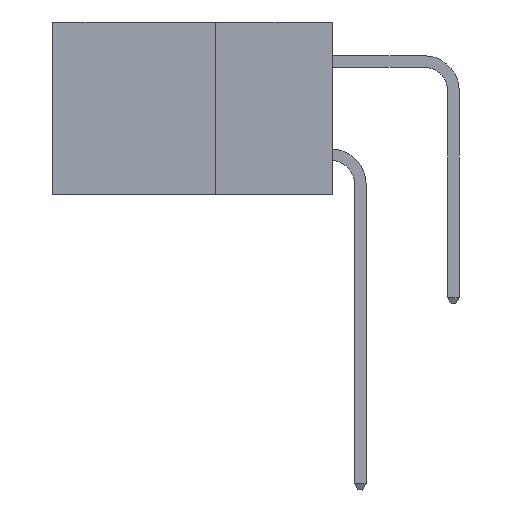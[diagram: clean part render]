
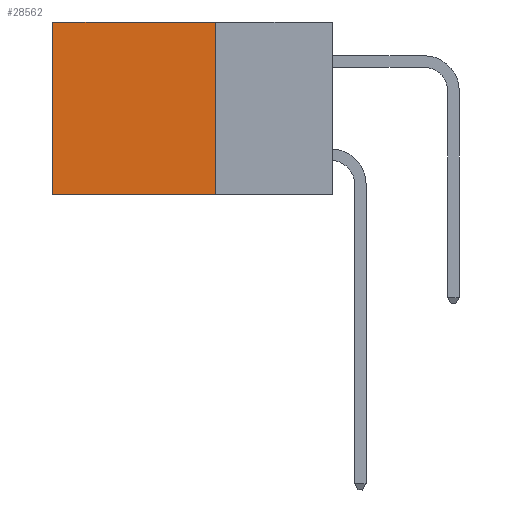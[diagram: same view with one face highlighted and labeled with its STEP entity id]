
A CAD part, left-side view. The second image highlights one B-rep face of the part: STEP entity #28562.
In plain terms, the highlighted planar face has unit normal (-1, 0, 0).
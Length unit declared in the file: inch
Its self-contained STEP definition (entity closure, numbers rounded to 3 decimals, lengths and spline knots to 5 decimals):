
#314 = DIRECTION ( 'NONE',  ( 0., 0., -1. ) ) ;
#470 = LINE ( 'NONE', #16206, #35874 ) ;
#710 = VERTEX_POINT ( 'NONE', #5032 ) ;
#717 = LINE ( 'NONE', #6351, #9896 ) ;
#2200 = DIRECTION ( 'NONE',  ( 0., 1., 0. ) ) ;
#3604 = ORIENTED_EDGE ( 'NONE', *, *, #19502, .F. ) ;
#4681 = VECTOR ( 'NONE', #33015, 39.37008 ) ;
#5032 = CARTESIAN_POINT ( 'NONE',  ( 0.298, 0.6, -0.37 ) ) ;
#5566 = LINE ( 'NONE', #13484, #4681 ) ;
#6351 = CARTESIAN_POINT ( 'NONE',  ( 0.298, 0.25, 0. ) ) ;
#9896 = VECTOR ( 'NONE', #25957, 39.37008 ) ;
#10123 = EDGE_CURVE ( 'NONE', #27809, #710, #29026, .T. ) ;
#10283 = EDGE_LOOP ( 'NONE', ( #22776, #3604, #24167, #32727 ) ) ;
#12335 = VERTEX_POINT ( 'NONE', #22253 ) ;
#13484 = CARTESIAN_POINT ( 'NONE',  ( 0.298, 0.25, 0. ) ) ;
#13722 = CARTESIAN_POINT ( 'NONE',  ( 0.298, 0.6, 0. ) ) ;
#14170 = VECTOR ( 'NONE', #16322, 39.37008 ) ;
#14858 = EDGE_CURVE ( 'NONE', #23234, #27809, #5566, .T. ) ;
#15185 = EDGE_CURVE ( 'NONE', #23234, #12335, #717, .T. ) ;
#16206 = CARTESIAN_POINT ( 'NONE',  ( 0.298, 0.25, -0.37 ) ) ;
#16322 = DIRECTION ( 'NONE',  ( 0., 0., -1. ) ) ;
#17132 = DIRECTION ( 'NONE',  ( 1., 0., 0. ) ) ;
#17193 = CARTESIAN_POINT ( 'NONE',  ( 0.298, 0.25, 0. ) ) ;
#19056 = AXIS2_PLACEMENT_3D ( 'NONE', #33801, #17132, #314 ) ;
#19502 = EDGE_CURVE ( 'NONE', #12335, #710, #470, .T. ) ;
#22253 = CARTESIAN_POINT ( 'NONE',  ( 0.298, 0.25, -0.37 ) ) ;
#22776 = ORIENTED_EDGE ( 'NONE', *, *, #10123, .T. ) ;
#23234 = VERTEX_POINT ( 'NONE', #17193 ) ;
#24167 = ORIENTED_EDGE ( 'NONE', *, *, #15185, .F. ) ;
#25439 = PLANE ( 'NONE',  #19056 ) ;
#25957 = DIRECTION ( 'NONE',  ( 0., 0., -1. ) ) ;
#26232 = FACE_OUTER_BOUND ( 'NONE', #10283, .T. ) ;
#27809 = VERTEX_POINT ( 'NONE', #13722 ) ;
#28562 = ADVANCED_FACE ( 'NONE', ( #26232 ), #25439, .F. ) ;
#29026 = LINE ( 'NONE', #30202, #14170 ) ;
#30202 = CARTESIAN_POINT ( 'NONE',  ( 0.298, 0.6, 0. ) ) ;
#32727 = ORIENTED_EDGE ( 'NONE', *, *, #14858, .T. ) ;
#33015 = DIRECTION ( 'NONE',  ( 0., 1., 0. ) ) ;
#33801 = CARTESIAN_POINT ( 'NONE',  ( 0.298, 0.25, 0. ) ) ;
#35874 = VECTOR ( 'NONE', #2200, 39.37008 ) ;
